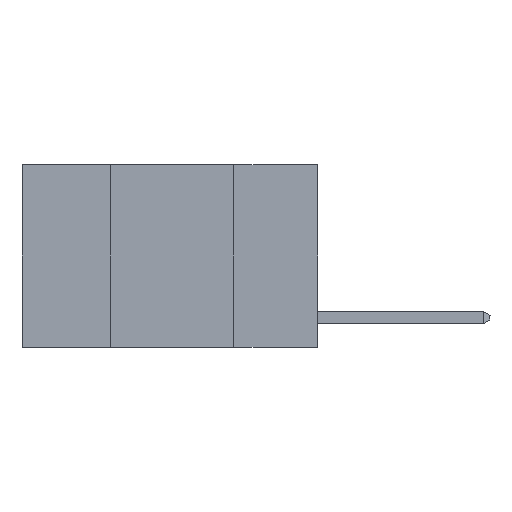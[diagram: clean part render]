
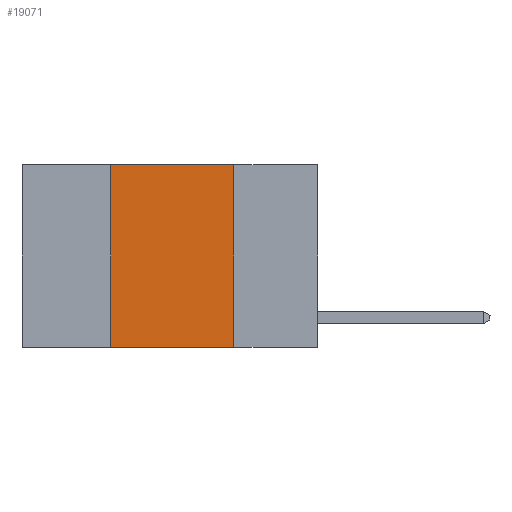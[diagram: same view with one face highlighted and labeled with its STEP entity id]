
A CAD part, left-side view. The second image highlights one B-rep face of the part: STEP entity #19071.
In plain terms, the highlighted planar face has unit normal (-1, 0, 0).
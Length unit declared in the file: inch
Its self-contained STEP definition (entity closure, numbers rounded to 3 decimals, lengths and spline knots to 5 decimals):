
#362 = AXIS2_PLACEMENT_3D ( 'NONE', #19559, #5213, #5553 ) ;
#609 = CARTESIAN_POINT ( 'NONE',  ( 0., 0.42, 0. ) ) ;
#639 = DIRECTION ( 'NONE',  ( 0., -1., 0. ) ) ;
#1652 = VERTEX_POINT ( 'NONE', #17001 ) ;
#2343 = LINE ( 'NONE', #609, #7017 ) ;
#2503 = EDGE_LOOP ( 'NONE', ( #7477, #14751, #19017, #19362 ) ) ;
#3355 = PLANE ( 'NONE',  #362 ) ;
#4099 = LINE ( 'NONE', #5610, #18265 ) ;
#4827 = EDGE_CURVE ( 'NONE', #14393, #12624, #9608, .T. ) ;
#4955 = CARTESIAN_POINT ( 'NONE',  ( 0., 0.42, -0.37 ) ) ;
#5213 = DIRECTION ( 'NONE',  ( 1., 0., 0. ) ) ;
#5553 = DIRECTION ( 'NONE',  ( 0., 0., -1. ) ) ;
#5610 = CARTESIAN_POINT ( 'NONE',  ( 0., 0.17, 0. ) ) ;
#5628 = LINE ( 'NONE', #12750, #17057 ) ;
#7017 = VECTOR ( 'NONE', #14805, 39.37008 ) ;
#7477 = ORIENTED_EDGE ( 'NONE', *, *, #20100, .F. ) ;
#7864 = CARTESIAN_POINT ( 'NONE',  ( 0., 0.6, 0. ) ) ;
#9608 = LINE ( 'NONE', #7864, #14169 ) ;
#11197 = DIRECTION ( 'NONE',  ( 0., 0., -1. ) ) ;
#12624 = VERTEX_POINT ( 'NONE', #14241 ) ;
#12750 = CARTESIAN_POINT ( 'NONE',  ( 0., 0.6, -0.37 ) ) ;
#14169 = VECTOR ( 'NONE', #18828, 39.37008 ) ;
#14241 = CARTESIAN_POINT ( 'NONE',  ( 0., 0.17, 0. ) ) ;
#14393 = VERTEX_POINT ( 'NONE', #19685 ) ;
#14751 = ORIENTED_EDGE ( 'NONE', *, *, #4827, .F. ) ;
#14805 = DIRECTION ( 'NONE',  ( 0., 0., 1. ) ) ;
#15332 = EDGE_CURVE ( 'NONE', #19383, #14393, #2343, .T. ) ;
#16170 = FACE_OUTER_BOUND ( 'NONE', #2503, .T. ) ;
#16569 = EDGE_CURVE ( 'NONE', #19383, #1652, #5628, .T. ) ;
#17001 = CARTESIAN_POINT ( 'NONE',  ( 0., 0.17, -0.37 ) ) ;
#17057 = VECTOR ( 'NONE', #639, 39.37008 ) ;
#18265 = VECTOR ( 'NONE', #11197, 39.37008 ) ;
#18828 = DIRECTION ( 'NONE',  ( 0., -1., 0. ) ) ;
#19017 = ORIENTED_EDGE ( 'NONE', *, *, #15332, .F. ) ;
#19071 = ADVANCED_FACE ( 'NONE', ( #16170 ), #3355, .F. ) ;
#19362 = ORIENTED_EDGE ( 'NONE', *, *, #16569, .T. ) ;
#19383 = VERTEX_POINT ( 'NONE', #4955 ) ;
#19559 = CARTESIAN_POINT ( 'NONE',  ( 0., 0.6, 0. ) ) ;
#19685 = CARTESIAN_POINT ( 'NONE',  ( 0., 0.42, 0. ) ) ;
#20100 = EDGE_CURVE ( 'NONE', #12624, #1652, #4099, .T. ) ;
